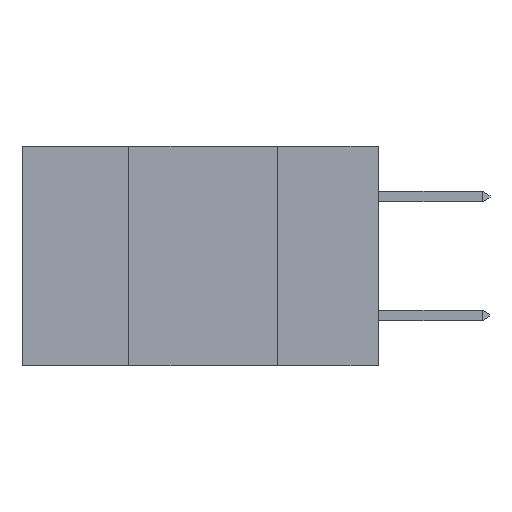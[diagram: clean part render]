
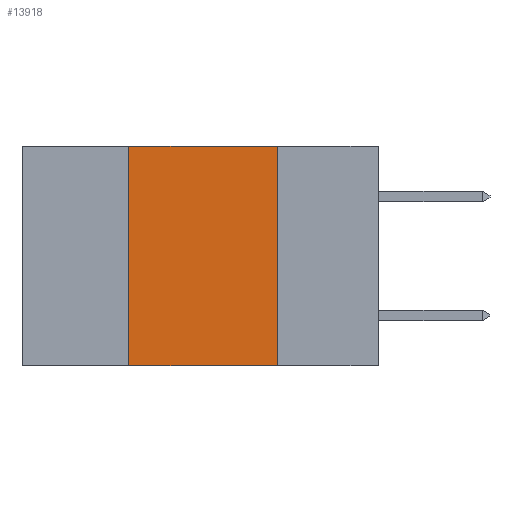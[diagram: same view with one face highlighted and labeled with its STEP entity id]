
A CAD part, left-side view. The second image highlights one B-rep face of the part: STEP entity #13918.
In plain terms, the highlighted planar face has unit normal (-1, 0, 0).
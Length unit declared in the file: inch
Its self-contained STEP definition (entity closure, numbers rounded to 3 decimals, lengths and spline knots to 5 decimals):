
#645 = CARTESIAN_POINT ( 'NONE',  ( 0., 0.17, 0. ) ) ;
#1878 = CARTESIAN_POINT ( 'NONE',  ( 0., 0.17, -0.37 ) ) ;
#1884 = AXIS2_PLACEMENT_3D ( 'NONE', #6947, #17981, #4842 ) ;
#2250 = CARTESIAN_POINT ( 'NONE',  ( 0., 0.6, 0. ) ) ;
#2590 = VERTEX_POINT ( 'NONE', #7178 ) ;
#2812 = DIRECTION ( 'NONE',  ( 0., 0., -1. ) ) ;
#4308 = LINE ( 'NONE', #2250, #15280 ) ;
#4675 = DIRECTION ( 'NONE',  ( 0., 0., 1. ) ) ;
#4842 = DIRECTION ( 'NONE',  ( 0., 0., -1. ) ) ;
#4937 = LINE ( 'NONE', #26308, #10104 ) ;
#5385 = ORIENTED_EDGE ( 'NONE', *, *, #8210, .T. ) ;
#6263 = VECTOR ( 'NONE', #2812, 39.37008 ) ;
#6738 = CARTESIAN_POINT ( 'NONE',  ( 0., 0.42, 0. ) ) ;
#6947 = CARTESIAN_POINT ( 'NONE',  ( 0., 0.6, 0. ) ) ;
#7178 = CARTESIAN_POINT ( 'NONE',  ( 0., 0.17, 0. ) ) ;
#8177 = VERTEX_POINT ( 'NONE', #19654 ) ;
#8210 = EDGE_CURVE ( 'NONE', #8177, #9479, #4937, .T. ) ;
#9178 = PLANE ( 'NONE',  #1884 ) ;
#9479 = VERTEX_POINT ( 'NONE', #1878 ) ;
#9732 = ORIENTED_EDGE ( 'NONE', *, *, #20602, .F. ) ;
#10104 = VECTOR ( 'NONE', #13216, 39.37008 ) ;
#12487 = LINE ( 'NONE', #26514, #23441 ) ;
#12799 = LINE ( 'NONE', #645, #6263 ) ;
#13216 = DIRECTION ( 'NONE',  ( 0., -1., 0. ) ) ;
#13918 = ADVANCED_FACE ( 'NONE', ( #19028 ), #9178, .F. ) ;
#14658 = EDGE_CURVE ( 'NONE', #2590, #9479, #12799, .T. ) ;
#15280 = VECTOR ( 'NONE', #24136, 39.37008 ) ;
#17981 = DIRECTION ( 'NONE',  ( 1., 0., 0. ) ) ;
#19028 = FACE_OUTER_BOUND ( 'NONE', #28092, .T. ) ;
#19654 = CARTESIAN_POINT ( 'NONE',  ( 0., 0.42, -0.37 ) ) ;
#20602 = EDGE_CURVE ( 'NONE', #24844, #2590, #4308, .T. ) ;
#21983 = EDGE_CURVE ( 'NONE', #8177, #24844, #12487, .T. ) ;
#23441 = VECTOR ( 'NONE', #4675, 39.37008 ) ;
#23451 = ORIENTED_EDGE ( 'NONE', *, *, #21983, .F. ) ;
#23855 = ORIENTED_EDGE ( 'NONE', *, *, #14658, .F. ) ;
#24136 = DIRECTION ( 'NONE',  ( 0., -1., 0. ) ) ;
#24844 = VERTEX_POINT ( 'NONE', #6738 ) ;
#26308 = CARTESIAN_POINT ( 'NONE',  ( 0., 0.6, -0.37 ) ) ;
#26514 = CARTESIAN_POINT ( 'NONE',  ( 0., 0.42, 0. ) ) ;
#28092 = EDGE_LOOP ( 'NONE', ( #23855, #9732, #23451, #5385 ) ) ;
